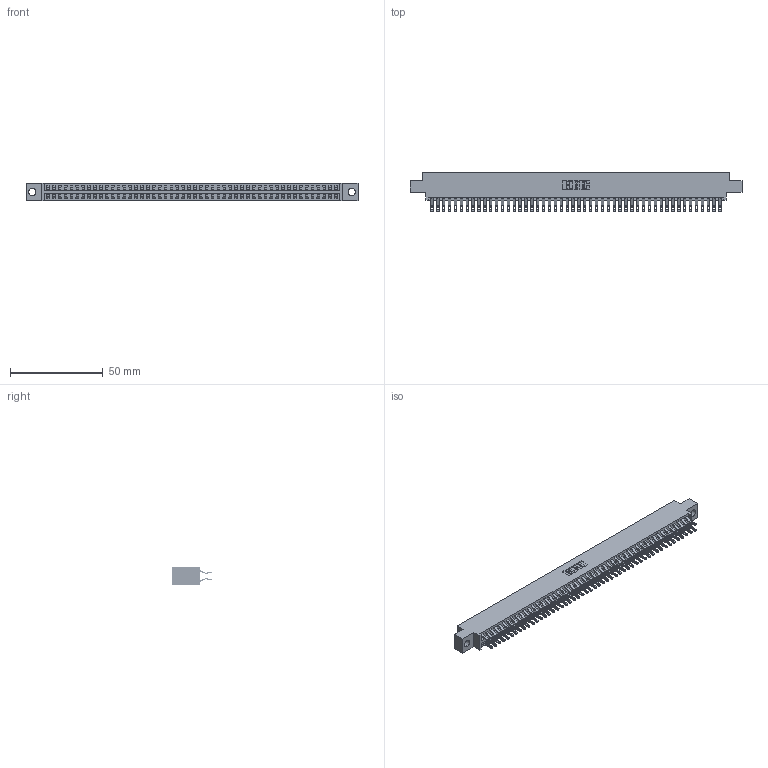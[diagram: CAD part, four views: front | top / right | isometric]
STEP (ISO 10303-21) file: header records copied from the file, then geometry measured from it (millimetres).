
FILE_DESCRIPTION (( 'STEP AP203' ), '1' );
FILE_NAME ('346-100-555-804.STEP', '2022-05-26T21:02:28', ( '' ), ( '' ), 'SwSTEP 2.0', 'SolidWorks 2020', '' );
FILE_SCHEMA (( 'CONFIG_CONTROL_DESIGN' ));
Length unit declared in the file: inch
Products named in the file (3): 345-292-001_555 Tail; 346 Part_0.170 Offset - 0.156 Dia-TH; 346-100-555-804
Assembly tree (101 placements, depth 2):
  346-100-555-804
    346 Part_0.170 Offset - 0.156 Dia-TH
    345-292-001_555 Tail  x100
Bounding box: 179.32 x 21.46 x 9.4 mm (x, y, z)
Volume: 17577.9 mm3; surface area: 25349.3 mm2
Topology: 101 solids, 101 shells, 5940 faces, 18677 edges, 12450 vertices
Faces by surface type: plane 3394, cylinder 2546
Entity records: 32431 total; most frequent: CARTESIAN_POINT 5376, ORIENTED_EDGE 5278, DIRECTION 4755, EDGE_CURVE 2639, LINE 2287, VECTOR 2287, VERTEX_POINT 1758, AXIS2_PLACEMENT_3D 1234
